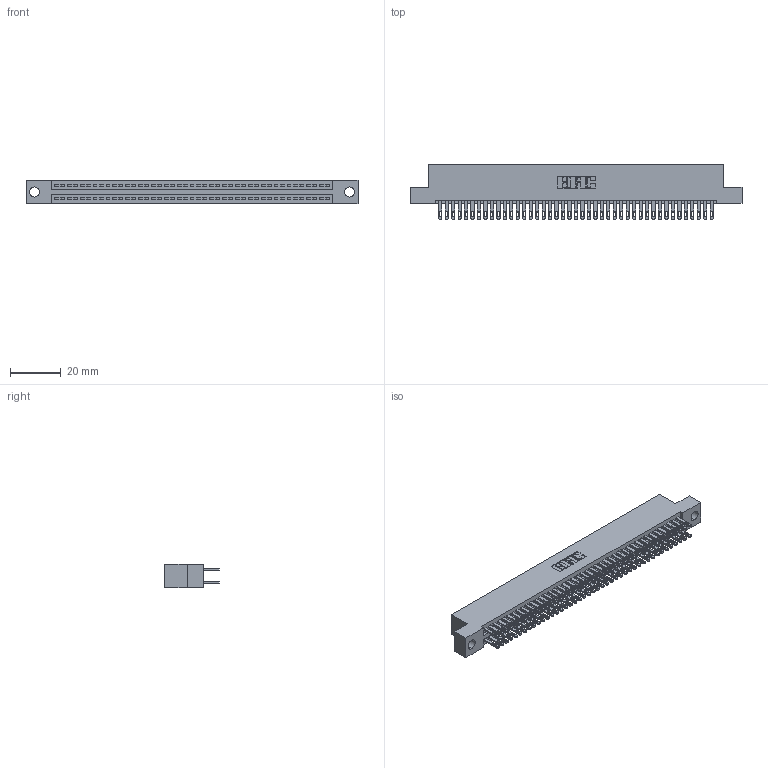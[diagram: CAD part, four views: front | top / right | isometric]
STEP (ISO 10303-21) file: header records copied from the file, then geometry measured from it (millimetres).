
FILE_DESCRIPTION (( 'STEP AP203' ), '1' );
FILE_NAME ('345-086-500-204.STEP', '2018-10-04T03:57:36', ( '' ), ( '' ), 'SwSTEP 2.0', 'SolidWorks 2016', '' );
FILE_SCHEMA (( 'CONFIG_CONTROL_DESIGN' ));
Length unit declared in the file: inch
Products named in the file (3): 345 Part_Flush Mounting Lugs - 0.156 Dia-TH; 345-292-001_345-293-100; 345-086-500-204
Assembly tree (87 placements, depth 2):
  345-086-500-204
    345 Part_Flush Mounting Lugs - 0.156 Dia-TH
    345-292-001_345-293-100  x86
Bounding box: 130.43 x 21.51 x 9.4 mm (x, y, z)
Volume: 12854.2 mm3; surface area: 19712.4 mm2
Topology: 87 solids, 87 shells, 4082 faces, 12467 edges, 8310 vertices
Faces by surface type: plane 2402, cylinder 1680
Entity records: 33537 total; most frequent: CARTESIAN_POINT 5620, ORIENTED_EDGE 5554, DIRECTION 4957, EDGE_CURVE 2777, LINE 2469, VECTOR 2469, VERTEX_POINT 1850, AXIS2_PLACEMENT_3D 1244
